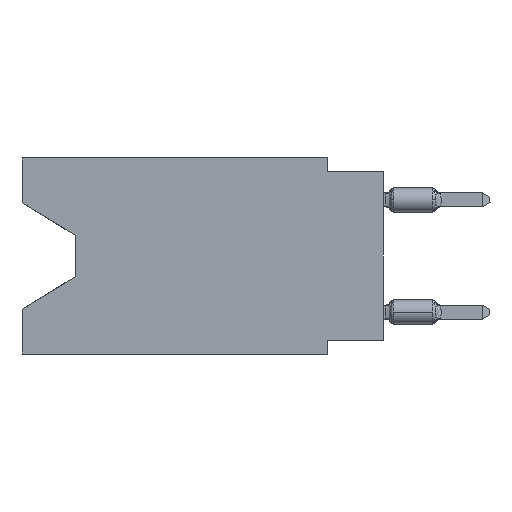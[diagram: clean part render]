
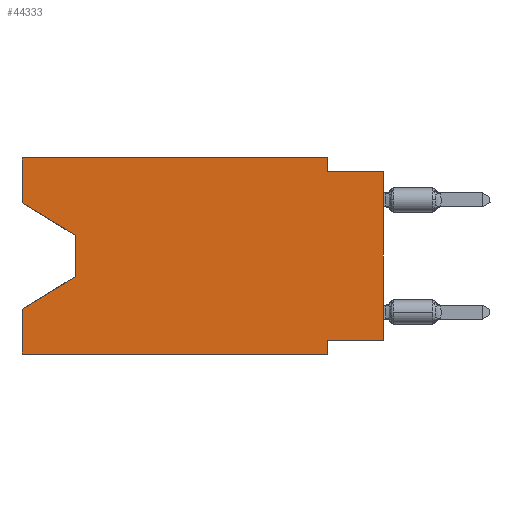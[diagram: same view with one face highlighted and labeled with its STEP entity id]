
A CAD part, left-side view. The second image highlights one B-rep face of the part: STEP entity #44333.
In plain terms, the highlighted planar face has unit normal (-1, 0, 0).
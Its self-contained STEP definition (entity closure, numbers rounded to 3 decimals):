
#215 = EDGE_CURVE ( 'NONE', #47082, #3216, #2268, .T. ) ;
#830 = DIRECTION ( 'NONE',  ( 0., -0.855, -0.519 ) ) ;
#903 = LINE ( 'NONE', #15449, #45340 ) ;
#938 = LINE ( 'NONE', #12849, #9156 ) ;
#1296 = VECTOR ( 'NONE', #32618, 1000. ) ;
#1552 = EDGE_CURVE ( 'NONE', #40197, #3216, #44305, .T. ) ;
#1647 = CARTESIAN_POINT ( 'NONE',  ( 0., 2.54, -0.635 ) ) ;
#2232 = VERTEX_POINT ( 'NONE', #26763 ) ;
#2268 = LINE ( 'NONE', #12989, #44829 ) ;
#2339 = ORIENTED_EDGE ( 'NONE', *, *, #3447, .F. ) ;
#2541 = CARTESIAN_POINT ( 'NONE',  ( 0., 16.383, -2.038 ) ) ;
#3068 = ORIENTED_EDGE ( 'NONE', *, *, #21179, .T. ) ;
#3173 = EDGE_CURVE ( 'NONE', #40197, #30744, #903, .T. ) ;
#3216 = VERTEX_POINT ( 'NONE', #38102 ) ;
#3447 = EDGE_CURVE ( 'NONE', #19076, #10636, #20948, .T. ) ;
#4246 = DIRECTION ( 'NONE',  ( 0., 0., 1. ) ) ;
#4519 = CARTESIAN_POINT ( 'NONE',  ( 0., 2.54, 0. ) ) ;
#4916 = DIRECTION ( 'NONE',  ( 0., 0., -1. ) ) ;
#6198 = EDGE_CURVE ( 'NONE', #44001, #2232, #8856, .T. ) ;
#6866 = LINE ( 'NONE', #28568, #1296 ) ;
#6940 = EDGE_CURVE ( 'NONE', #2232, #30744, #13431, .T. ) ;
#8856 = LINE ( 'NONE', #16269, #14327 ) ;
#9000 = CARTESIAN_POINT ( 'NONE',  ( 0., 2.54, 0. ) ) ;
#9156 = VECTOR ( 'NONE', #30029, 1000. ) ;
#9512 = DIRECTION ( 'NONE',  ( 0., -1., 0. ) ) ;
#10636 = VERTEX_POINT ( 'NONE', #21181 ) ;
#10982 = LINE ( 'NONE', #32685, #31071 ) ;
#11114 = VERTEX_POINT ( 'NONE', #2541 ) ;
#11210 = CARTESIAN_POINT ( 'NONE',  ( 0., 13.97, -3.505 ) ) ;
#12849 = CARTESIAN_POINT ( 'NONE',  ( 0., 13.97, -3.505 ) ) ;
#12989 = CARTESIAN_POINT ( 'NONE',  ( 0., 13.97, -5.385 ) ) ;
#13431 = LINE ( 'NONE', #16807, #20686 ) ;
#14307 = DIRECTION ( 'NONE',  ( 0., 0., 1. ) ) ;
#14327 = VECTOR ( 'NONE', #19584, 1000. ) ;
#14477 = ORIENTED_EDGE ( 'NONE', *, *, #6940, .F. ) ;
#14650 = ORIENTED_EDGE ( 'NONE', *, *, #40279, .F. ) ;
#15449 = CARTESIAN_POINT ( 'NONE',  ( 0., 16.383, -8.89 ) ) ;
#15929 = EDGE_CURVE ( 'NONE', #44001, #10636, #6866, .T. ) ;
#16269 = CARTESIAN_POINT ( 'NONE',  ( 0., 0., -8.255 ) ) ;
#16807 = CARTESIAN_POINT ( 'NONE',  ( 0., 2.54, -8.89 ) ) ;
#17487 = ORIENTED_EDGE ( 'NONE', *, *, #17976, .T. ) ;
#17499 = EDGE_CURVE ( 'NONE', #30831, #47141, #38082, .T. ) ;
#17976 = EDGE_CURVE ( 'NONE', #11114, #37126, #19179, .T. ) ;
#18564 = ORIENTED_EDGE ( 'NONE', *, *, #6198, .F. ) ;
#19076 = VERTEX_POINT ( 'NONE', #1647 ) ;
#19179 = LINE ( 'NONE', #41359, #37674 ) ;
#19498 = VECTOR ( 'NONE', #9512, 1000. ) ;
#19584 = DIRECTION ( 'NONE',  ( 0., 1., 0. ) ) ;
#19702 = VECTOR ( 'NONE', #4246, 1000. ) ;
#20686 = VECTOR ( 'NONE', #31098, 1000. ) ;
#20711 = CARTESIAN_POINT ( 'NONE',  ( 0., 0., -0.635 ) ) ;
#20948 = LINE ( 'NONE', #20711, #19498 ) ;
#21179 = EDGE_CURVE ( 'NONE', #37126, #47082, #938, .T. ) ;
#21181 = CARTESIAN_POINT ( 'NONE',  ( 0., 0., -0.635 ) ) ;
#22559 = FACE_OUTER_BOUND ( 'NONE', #42488, .T. ) ;
#22877 = CARTESIAN_POINT ( 'NONE',  ( 0., 13.97, -5.385 ) ) ;
#26380 = DIRECTION ( 'NONE',  ( 0., -1., 0. ) ) ;
#26763 = CARTESIAN_POINT ( 'NONE',  ( 0., 2.54, -8.255 ) ) ;
#26925 = ORIENTED_EDGE ( 'NONE', *, *, #1552, .F. ) ;
#27542 = DIRECTION ( 'NONE',  ( 0., 0.855, -0.519 ) ) ;
#28568 = CARTESIAN_POINT ( 'NONE',  ( 0., 0., 0. ) ) ;
#28843 = VECTOR ( 'NONE', #30938, 1000. ) ;
#29489 = DIRECTION ( 'NONE',  ( 1., 0., 0. ) ) ;
#29961 = CARTESIAN_POINT ( 'NONE',  ( 0., 16.383, 0. ) ) ;
#30029 = DIRECTION ( 'NONE',  ( 0., 0., -1. ) ) ;
#30744 = VERTEX_POINT ( 'NONE', #41667 ) ;
#30831 = VERTEX_POINT ( 'NONE', #34747 ) ;
#30938 = DIRECTION ( 'NONE',  ( 0., 0., -1. ) ) ;
#31071 = VECTOR ( 'NONE', #14307, 1000. ) ;
#31098 = DIRECTION ( 'NONE',  ( 0., 0., -1. ) ) ;
#31232 = ORIENTED_EDGE ( 'NONE', *, *, #46966, .F. ) ;
#31381 = AXIS2_PLACEMENT_3D ( 'NONE', #29961, #29489, #4916 ) ;
#31410 = ORIENTED_EDGE ( 'NONE', *, *, #215, .T. ) ;
#32618 = DIRECTION ( 'NONE',  ( 0., 0., 1. ) ) ;
#32685 = CARTESIAN_POINT ( 'NONE',  ( 0., 16.383, 0. ) ) ;
#33072 = PLANE ( 'NONE',  #31381 ) ;
#34747 = CARTESIAN_POINT ( 'NONE',  ( 0., 16.383, 0. ) ) ;
#35686 = VECTOR ( 'NONE', #26380, 1000. ) ;
#36125 = ORIENTED_EDGE ( 'NONE', *, *, #17499, .F. ) ;
#37126 = VERTEX_POINT ( 'NONE', #11210 ) ;
#37346 = ORIENTED_EDGE ( 'NONE', *, *, #3173, .T. ) ;
#37674 = VECTOR ( 'NONE', #830, 1000. ) ;
#38082 = LINE ( 'NONE', #44730, #35686 ) ;
#38102 = CARTESIAN_POINT ( 'NONE',  ( 0., 16.383, -6.852 ) ) ;
#40197 = VERTEX_POINT ( 'NONE', #43442 ) ;
#40279 = EDGE_CURVE ( 'NONE', #47141, #19076, #42160, .T. ) ;
#41359 = CARTESIAN_POINT ( 'NONE',  ( 0., 16.383, -2.038 ) ) ;
#41430 = DIRECTION ( 'NONE',  ( 0., -1., 0. ) ) ;
#41667 = CARTESIAN_POINT ( 'NONE',  ( 0., 2.54, -8.89 ) ) ;
#42160 = LINE ( 'NONE', #9000, #28843 ) ;
#42488 = EDGE_LOOP ( 'NONE', ( #17487, #3068, #31410, #26925, #37346, #14477, #18564, #46674, #2339, #14650, #36125, #31232 ) ) ;
#43442 = CARTESIAN_POINT ( 'NONE',  ( 0., 16.383, -8.89 ) ) ;
#43836 = CARTESIAN_POINT ( 'NONE',  ( 0., 16.383, 0. ) ) ;
#44001 = VERTEX_POINT ( 'NONE', #44783 ) ;
#44305 = LINE ( 'NONE', #43836, #19702 ) ;
#44333 = ADVANCED_FACE ( 'NONE', ( #22559 ), #33072, .F. ) ;
#44730 = CARTESIAN_POINT ( 'NONE',  ( 0., 16.383, 0. ) ) ;
#44783 = CARTESIAN_POINT ( 'NONE',  ( 0., 0., -8.255 ) ) ;
#44829 = VECTOR ( 'NONE', #27542, 1000. ) ;
#45340 = VECTOR ( 'NONE', #41430, 1000. ) ;
#46674 = ORIENTED_EDGE ( 'NONE', *, *, #15929, .T. ) ;
#46966 = EDGE_CURVE ( 'NONE', #11114, #30831, #10982, .T. ) ;
#47082 = VERTEX_POINT ( 'NONE', #22877 ) ;
#47141 = VERTEX_POINT ( 'NONE', #4519 ) ;
